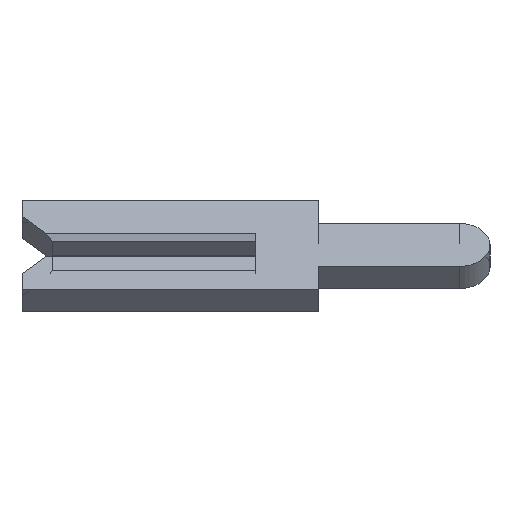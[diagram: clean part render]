
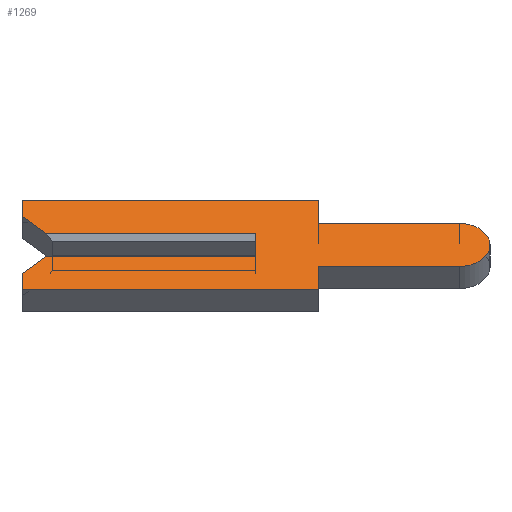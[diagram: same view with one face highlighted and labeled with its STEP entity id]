
A CAD part, left-side view. The second image highlights one B-rep face of the part: STEP entity #1269.
In plain terms, the highlighted face is planar.
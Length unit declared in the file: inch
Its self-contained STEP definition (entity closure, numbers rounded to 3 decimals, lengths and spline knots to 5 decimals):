
#1 = CARTESIAN_POINT ( 'NONE',  ( -0.01, 0.15, 0.026 ) ) ;
#24 = CARTESIAN_POINT ( 'NONE',  ( -0.01, 0.1305, -0.0065 ) ) ;
#52 = DIRECTION ( 'NONE',  ( 1., 0., 0. ) ) ;
#82 = DIRECTION ( 'NONE',  ( 0., 0.707, 0.707 ) ) ;
#86 = VECTOR ( 'NONE', #1443, 39.37008 ) ;
#116 = VERTEX_POINT ( 'NONE', #1587 ) ;
#137 = EDGE_CURVE ( 'NONE', #1091, #1578, #937, .T. ) ;
#156 = VERTEX_POINT ( 'NONE', #1284 ) ;
#159 = VERTEX_POINT ( 'NONE', #734 ) ;
#173 = CARTESIAN_POINT ( 'NONE',  ( -0.01, 0., -0.01 ) ) ;
#181 = CARTESIAN_POINT ( 'NONE',  ( -0.01, 0.15, 0.04 ) ) ;
#198 = DIRECTION ( 'NONE',  ( 0., -1., 0. ) ) ;
#215 = LINE ( 'NONE', #589, #890 ) ;
#224 = VERTEX_POINT ( 'NONE', #173 ) ;
#242 = ORIENTED_EDGE ( 'NONE', *, *, #868, .F. ) ;
#256 = ORIENTED_EDGE ( 'NONE', *, *, #453, .T. ) ;
#257 = DIRECTION ( 'NONE',  ( 0., 1., 0. ) ) ;
#292 = EDGE_LOOP ( 'NONE', ( #256, #1290, #1011, #965, #242, #1415, #1216, #314, #1695, #1801, #1678, #302, #953, #676 ) ) ;
#302 = ORIENTED_EDGE ( 'NONE', *, *, #697, .F. ) ;
#314 = ORIENTED_EDGE ( 'NONE', *, *, #1095, .F. ) ;
#337 = FACE_OUTER_BOUND ( 'NONE', #292, .T. ) ;
#367 = DIRECTION ( 'NONE',  ( 0., 0., -1. ) ) ;
#375 = DIRECTION ( 'NONE',  ( 0., -1., 0. ) ) ;
#422 = CARTESIAN_POINT ( 'NONE',  ( -0.01, 0.15, 0.04 ) ) ;
#444 = CARTESIAN_POINT ( 'NONE',  ( -0.01, -0.04, -0.04 ) ) ;
#453 = EDGE_CURVE ( 'NONE', #464, #1354, #215, .T. ) ;
#464 = VERTEX_POINT ( 'NONE', #1194 ) ;
#468 = DIRECTION ( 'NONE',  ( 0., -1., 0. ) ) ;
#496 = DIRECTION ( 'NONE',  ( 0., 0., -1. ) ) ;
#580 = DIRECTION ( 'NONE',  ( 0., 0., 1. ) ) ;
#589 = CARTESIAN_POINT ( 'NONE',  ( -0.01, 0.15, 0.01 ) ) ;
#593 = VERTEX_POINT ( 'NONE', #1339 ) ;
#595 = VECTOR ( 'NONE', #257, 39.37008 ) ;
#598 = LINE ( 'NONE', #1520, #1467 ) ;
#645 = LINE ( 'NONE', #785, #1369 ) ;
#676 = ORIENTED_EDGE ( 'NONE', *, *, #1325, .F. ) ;
#686 = VECTOR ( 'NONE', #968, 39.37008 ) ;
#696 = CARTESIAN_POINT ( 'NONE',  ( -0.01, -0.1305, -0.01 ) ) ;
#697 = EDGE_CURVE ( 'NONE', #1578, #116, #1810, .T. ) ;
#706 = LINE ( 'NONE', #696, #1005 ) ;
#734 = CARTESIAN_POINT ( 'NONE',  ( -0.01, -0.04, -0.04 ) ) ;
#768 = CARTESIAN_POINT ( 'NONE',  ( -0.01, -0.1305, 0. ) ) ;
#770 = VECTOR ( 'NONE', #367, 39.37008 ) ;
#781 = DIRECTION ( 'NONE',  ( 0., -1., 0. ) ) ;
#785 = CARTESIAN_POINT ( 'NONE',  ( -0.01, 0.15, -0.026 ) ) ;
#798 = VERTEX_POINT ( 'NONE', #921 ) ;
#800 = EDGE_CURVE ( 'NONE', #1646, #843, #598, .T. ) ;
#804 = CARTESIAN_POINT ( 'NONE',  ( -0.01, 0., 0.01 ) ) ;
#823 = LINE ( 'NONE', #961, #595 ) ;
#843 = VERTEX_POINT ( 'NONE', #1812 ) ;
#848 = CARTESIAN_POINT ( 'NONE',  ( -0.01, -0.04, 0.0195 ) ) ;
#868 = EDGE_CURVE ( 'NONE', #1170, #593, #645, .T. ) ;
#890 = VECTOR ( 'NONE', #468, 39.37008 ) ;
#904 = EDGE_CURVE ( 'NONE', #843, #1465, #1031, .T. ) ;
#921 = CARTESIAN_POINT ( 'NONE',  ( -0.01, 0.134, -0.01 ) ) ;
#937 = LINE ( 'NONE', #1745, #1304 ) ;
#945 = CARTESIAN_POINT ( 'NONE',  ( -0.01, 0.1305, 0.0065 ) ) ;
#953 = ORIENTED_EDGE ( 'NONE', *, *, #137, .F. ) ;
#961 = CARTESIAN_POINT ( 'NONE',  ( -0.01, -0.04, -0.0195 ) ) ;
#962 = VECTOR ( 'NONE', #1317, 39.37008 ) ;
#964 = LINE ( 'NONE', #1372, #686 ) ;
#965 = ORIENTED_EDGE ( 'NONE', *, *, #1620, .F. ) ;
#968 = DIRECTION ( 'NONE',  ( 0., 0., 1. ) ) ;
#1005 = VECTOR ( 'NONE', #375, 39.37008 ) ;
#1011 = ORIENTED_EDGE ( 'NONE', *, *, #1693, .F. ) ;
#1031 = CIRCLE ( 'NONE', #1077, 0.0195 ) ;
#1077 = AXIS2_PLACEMENT_3D ( 'NONE', #768, #52, #496 ) ;
#1091 = VERTEX_POINT ( 'NONE', #1 ) ;
#1095 = EDGE_CURVE ( 'NONE', #1465, #156, #823, .T. ) ;
#1104 = AXIS2_PLACEMENT_3D ( 'NONE', #1247, #1696, #1109 ) ;
#1109 = DIRECTION ( 'NONE',  ( 0., 0., -1. ) ) ;
#1122 = LINE ( 'NONE', #1262, #770 ) ;
#1135 = CARTESIAN_POINT ( 'NONE',  ( -0.01, -0.1305, -0.0195 ) ) ;
#1169 = EDGE_CURVE ( 'NONE', #116, #1646, #1122, .T. ) ;
#1170 = VERTEX_POINT ( 'NONE', #1306 ) ;
#1194 = CARTESIAN_POINT ( 'NONE',  ( -0.01, 0.134, 0.01 ) ) ;
#1213 = LINE ( 'NONE', #1736, #1834 ) ;
#1216 = ORIENTED_EDGE ( 'NONE', *, *, #1785, .F. ) ;
#1247 = CARTESIAN_POINT ( 'NONE',  ( -0.01, -0.1305, 0. ) ) ;
#1262 = CARTESIAN_POINT ( 'NONE',  ( -0.01, -0.04, 0.04 ) ) ;
#1269 = ADVANCED_FACE ( 'NONE', ( #337 ), #1390, .F. ) ;
#1284 = CARTESIAN_POINT ( 'NONE',  ( -0.01, -0.04, -0.0195 ) ) ;
#1290 = ORIENTED_EDGE ( 'NONE', *, *, #1425, .F. ) ;
#1301 = LINE ( 'NONE', #444, #962 ) ;
#1304 = VECTOR ( 'NONE', #580, 39.37008 ) ;
#1306 = CARTESIAN_POINT ( 'NONE',  ( -0.01, 0.15, -0.04 ) ) ;
#1317 = DIRECTION ( 'NONE',  ( 0., 0., -1. ) ) ;
#1325 = EDGE_CURVE ( 'NONE', #464, #1091, #1437, .T. ) ;
#1339 = CARTESIAN_POINT ( 'NONE',  ( -0.01, 0.15, -0.026 ) ) ;
#1348 = VECTOR ( 'NONE', #82, 39.37008 ) ;
#1354 = VERTEX_POINT ( 'NONE', #804 ) ;
#1369 = VECTOR ( 'NONE', #1371, 39.37008 ) ;
#1371 = DIRECTION ( 'NONE',  ( 0., 0., 1. ) ) ;
#1372 = CARTESIAN_POINT ( 'NONE',  ( -0.01, 0., 0.0065 ) ) ;
#1390 = PLANE ( 'NONE',  #1104 ) ;
#1415 = ORIENTED_EDGE ( 'NONE', *, *, #1819, .F. ) ;
#1425 = EDGE_CURVE ( 'NONE', #224, #1354, #964, .T. ) ;
#1437 = LINE ( 'NONE', #945, #1348 ) ;
#1443 = DIRECTION ( 'NONE',  ( 0., -0.707, 0.707 ) ) ;
#1465 = VERTEX_POINT ( 'NONE', #1135 ) ;
#1467 = VECTOR ( 'NONE', #781, 39.37008 ) ;
#1486 = LINE ( 'NONE', #24, #86 ) ;
#1520 = CARTESIAN_POINT ( 'NONE',  ( -0.01, -0.04, 0.0195 ) ) ;
#1578 = VERTEX_POINT ( 'NONE', #422 ) ;
#1587 = CARTESIAN_POINT ( 'NONE',  ( -0.01, -0.04, 0.04 ) ) ;
#1620 = EDGE_CURVE ( 'NONE', #593, #798, #1486, .T. ) ;
#1646 = VERTEX_POINT ( 'NONE', #848 ) ;
#1678 = ORIENTED_EDGE ( 'NONE', *, *, #1169, .F. ) ;
#1693 = EDGE_CURVE ( 'NONE', #798, #224, #706, .T. ) ;
#1695 = ORIENTED_EDGE ( 'NONE', *, *, #904, .F. ) ;
#1696 = DIRECTION ( 'NONE',  ( 1., 0., 0. ) ) ;
#1697 = VECTOR ( 'NONE', #198, 39.37008 ) ;
#1728 = DIRECTION ( 'NONE',  ( 0., 1., 0. ) ) ;
#1736 = CARTESIAN_POINT ( 'NONE',  ( -0.01, 0.15, -0.04 ) ) ;
#1745 = CARTESIAN_POINT ( 'NONE',  ( -0.01, 0.15, 0.026 ) ) ;
#1785 = EDGE_CURVE ( 'NONE', #156, #159, #1301, .T. ) ;
#1801 = ORIENTED_EDGE ( 'NONE', *, *, #800, .F. ) ;
#1810 = LINE ( 'NONE', #181, #1697 ) ;
#1812 = CARTESIAN_POINT ( 'NONE',  ( -0.01, -0.1305, 0.0195 ) ) ;
#1819 = EDGE_CURVE ( 'NONE', #159, #1170, #1213, .T. ) ;
#1834 = VECTOR ( 'NONE', #1728, 39.37008 ) ;
